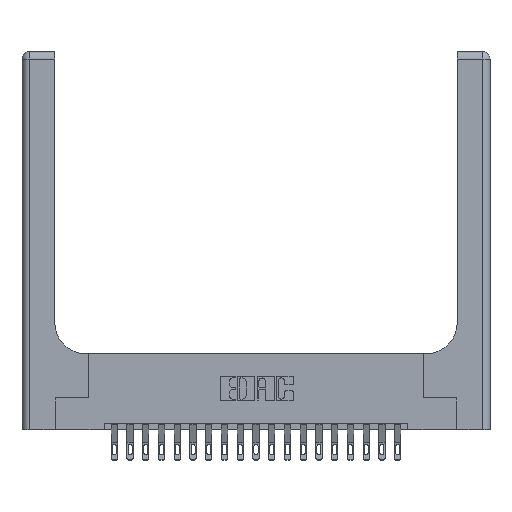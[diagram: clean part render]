
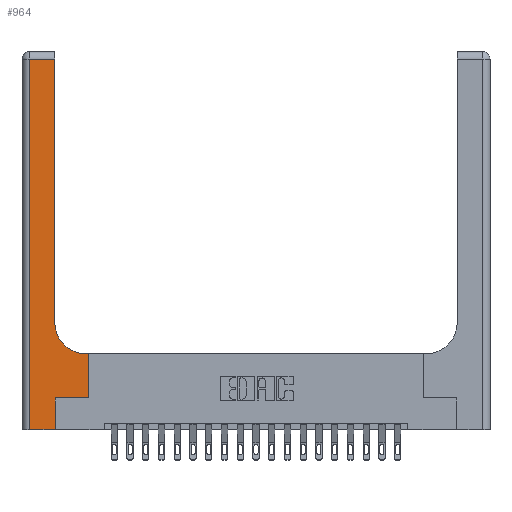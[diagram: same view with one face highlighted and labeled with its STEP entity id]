
A CAD part, top view. The second image highlights one B-rep face of the part: STEP entity #964.
In plain terms, the highlighted planar face has unit normal (0, 0, 1).
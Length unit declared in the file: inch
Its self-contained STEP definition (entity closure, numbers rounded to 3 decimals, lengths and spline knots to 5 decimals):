
#8 = ORIENTED_EDGE ( 'NONE', *, *, #1246, .T. ) ;
#551 = VECTOR ( 'NONE', #1694, 39.37008 ) ;
#736 = CARTESIAN_POINT ( 'NONE',  ( 0.51, 0.85, 0.37 ) ) ;
#803 = CARTESIAN_POINT ( 'NONE',  ( 0.51, 0.6, 0.37 ) ) ;
#857 = LINE ( 'NONE', #14228, #7415 ) ;
#964 = ADVANCED_FACE ( 'NONE', ( #18222 ), #11533, .F. ) ;
#1246 = EDGE_CURVE ( 'NONE', #11904, #7707, #18068, .T. ) ;
#1694 = DIRECTION ( 'NONE',  ( 0., -1., 0. ) ) ;
#2240 = DIRECTION ( 'NONE',  ( 0., 0., -1. ) ) ;
#2287 = VECTOR ( 'NONE', #6582, 39.37008 ) ;
#2391 = CARTESIAN_POINT ( 'NONE',  ( 0.26, 3., 0.37 ) ) ;
#2403 = VECTOR ( 'NONE', #20437, 39.37008 ) ;
#3160 = CARTESIAN_POINT ( 'NONE',  ( 0., 3., 0.37 ) ) ;
#3461 = CARTESIAN_POINT ( 'NONE',  ( 0.528, 0.6, 0.37 ) ) ;
#3653 = EDGE_CURVE ( 'NONE', #4183, #5835, #4033, .T. ) ;
#3881 = DIRECTION ( 'NONE',  ( -1., 0., 0. ) ) ;
#4033 = LINE ( 'NONE', #2391, #16476 ) ;
#4060 = EDGE_CURVE ( 'NONE', #11592, #4183, #20649, .T. ) ;
#4183 = VERTEX_POINT ( 'NONE', #19174 ) ;
#4389 = ORIENTED_EDGE ( 'NONE', *, *, #16139, .T. ) ;
#4629 = ORIENTED_EDGE ( 'NONE', *, *, #14815, .T. ) ;
#5378 = LINE ( 'NONE', #13857, #2403 ) ;
#5835 = VERTEX_POINT ( 'NONE', #7116 ) ;
#5962 = VECTOR ( 'NONE', #10052, 39.37008 ) ;
#6582 = DIRECTION ( 'NONE',  ( 1., 0., 0. ) ) ;
#6871 = DIRECTION ( 'NONE',  ( -1., 0., 0. ) ) ;
#7116 = CARTESIAN_POINT ( 'NONE',  ( 0.26, 2.94, 0.37 ) ) ;
#7194 = EDGE_LOOP ( 'NONE', ( #8350, #4629, #8, #21252, #12591, #18813, #11773, #4389, #19562 ) ) ;
#7266 = LINE ( 'NONE', #8381, #11963 ) ;
#7415 = VECTOR ( 'NONE', #7619, 39.37008 ) ;
#7619 = DIRECTION ( 'NONE',  ( -1., 0., 0. ) ) ;
#7707 = VERTEX_POINT ( 'NONE', #14344 ) ;
#8183 = AXIS2_PLACEMENT_3D ( 'NONE', #3160, #2240, #6871 ) ;
#8350 = ORIENTED_EDGE ( 'NONE', *, *, #3653, .T. ) ;
#8381 = CARTESIAN_POINT ( 'NONE',  ( 0., 2.94, 0.37 ) ) ;
#9417 = VERTEX_POINT ( 'NONE', #9631 ) ;
#9566 = EDGE_CURVE ( 'NONE', #11836, #9417, #5378, .T. ) ;
#9631 = CARTESIAN_POINT ( 'NONE',  ( 0.265, 0.25, 0.37 ) ) ;
#9916 = CARTESIAN_POINT ( 'NONE',  ( 0.265, 0., 0.37 ) ) ;
#10052 = DIRECTION ( 'NONE',  ( 0., 1., 0. ) ) ;
#10463 = VECTOR ( 'NONE', #13842, 39.37008 ) ;
#11318 = AXIS2_PLACEMENT_3D ( 'NONE', #736, #13907, #13584 ) ;
#11424 = EDGE_CURVE ( 'NONE', #20682, #16467, #14947, .T. ) ;
#11533 = PLANE ( 'NONE',  #8183 ) ;
#11587 = CARTESIAN_POINT ( 'NONE',  ( 0.528, 0.25, 0.37 ) ) ;
#11592 = VERTEX_POINT ( 'NONE', #803 ) ;
#11773 = ORIENTED_EDGE ( 'NONE', *, *, #11424, .T. ) ;
#11816 = CARTESIAN_POINT ( 'NONE',  ( 0.06, 3., 0.37 ) ) ;
#11836 = VERTEX_POINT ( 'NONE', #9916 ) ;
#11904 = VERTEX_POINT ( 'NONE', #20530 ) ;
#11963 = VECTOR ( 'NONE', #3881, 39.37008 ) ;
#11998 = EDGE_CURVE ( 'NONE', #9417, #20682, #14050, .T. ) ;
#12591 = ORIENTED_EDGE ( 'NONE', *, *, #9566, .T. ) ;
#13584 = DIRECTION ( 'NONE',  ( 1., 0., 0. ) ) ;
#13842 = DIRECTION ( 'NONE',  ( 1., 0., 0. ) ) ;
#13857 = CARTESIAN_POINT ( 'NONE',  ( 0.265, 0., 0.37 ) ) ;
#13907 = DIRECTION ( 'NONE',  ( 0., 0., -1. ) ) ;
#14050 = LINE ( 'NONE', #18679, #10463 ) ;
#14228 = CARTESIAN_POINT ( 'NONE',  ( 0.26, 0.6, 0.37 ) ) ;
#14344 = CARTESIAN_POINT ( 'NONE',  ( 0.06, 0., 0.37 ) ) ;
#14815 = EDGE_CURVE ( 'NONE', #5835, #11904, #7266, .T. ) ;
#14947 = LINE ( 'NONE', #11587, #5962 ) ;
#16139 = EDGE_CURVE ( 'NONE', #16467, #11592, #857, .T. ) ;
#16234 = LINE ( 'NONE', #18151, #2287 ) ;
#16467 = VERTEX_POINT ( 'NONE', #3461 ) ;
#16476 = VECTOR ( 'NONE', #17469, 39.37008 ) ;
#17469 = DIRECTION ( 'NONE',  ( 0., 1., 0. ) ) ;
#17922 = CARTESIAN_POINT ( 'NONE',  ( 0.528, 0.25, 0.37 ) ) ;
#18068 = LINE ( 'NONE', #11816, #551 ) ;
#18151 = CARTESIAN_POINT ( 'NONE',  ( 0., 0., 0.37 ) ) ;
#18222 = FACE_OUTER_BOUND ( 'NONE', #7194, .T. ) ;
#18679 = CARTESIAN_POINT ( 'NONE',  ( 0.265, 0.25, 0.37 ) ) ;
#18813 = ORIENTED_EDGE ( 'NONE', *, *, #11998, .T. ) ;
#19174 = CARTESIAN_POINT ( 'NONE',  ( 0.26, 0.85, 0.37 ) ) ;
#19243 = EDGE_CURVE ( 'NONE', #7707, #11836, #16234, .T. ) ;
#19562 = ORIENTED_EDGE ( 'NONE', *, *, #4060, .T. ) ;
#20437 = DIRECTION ( 'NONE',  ( 0., 1., 0. ) ) ;
#20530 = CARTESIAN_POINT ( 'NONE',  ( 0.06, 2.94, 0.37 ) ) ;
#20649 = CIRCLE ( 'NONE', #11318, 0.25 ) ;
#20682 = VERTEX_POINT ( 'NONE', #17922 ) ;
#21252 = ORIENTED_EDGE ( 'NONE', *, *, #19243, .T. ) ;
